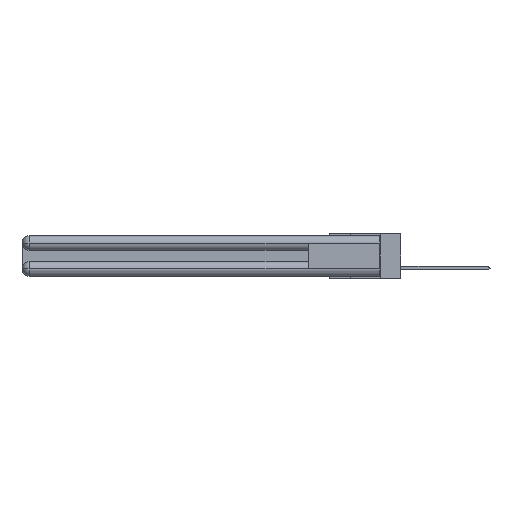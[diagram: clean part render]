
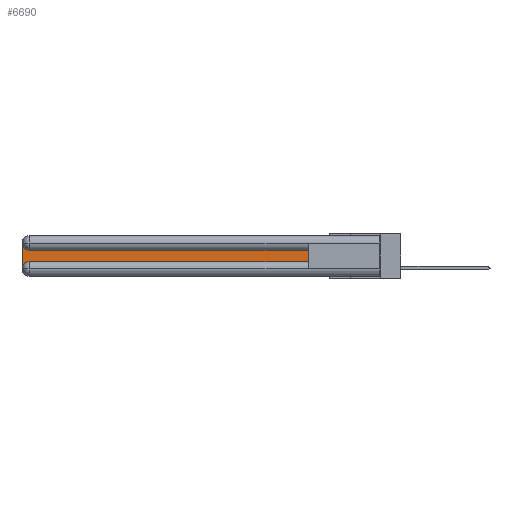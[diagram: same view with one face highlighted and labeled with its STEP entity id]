
A CAD part, left-side view. The second image highlights one B-rep face of the part: STEP entity #6690.
In plain terms, the highlighted planar face has unit normal (-1, 0, 0).
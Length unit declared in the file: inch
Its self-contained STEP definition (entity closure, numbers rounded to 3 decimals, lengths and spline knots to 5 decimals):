
#36 = LINE ( 'NONE', #24860, #5275 ) ;
#130 = EDGE_LOOP ( 'NONE', ( #14637, #1861, #14647, #15981, #6974, #20860 ) ) ;
#1607 = DIRECTION ( 'NONE',  ( 0., 0., -1. ) ) ;
#1852 = CARTESIAN_POINT ( 'NONE',  ( 0.075, 2.94, -0.1225 ) ) ;
#1861 = ORIENTED_EDGE ( 'NONE', *, *, #5569, .T. ) ;
#3278 = VERTEX_POINT ( 'NONE', #14300 ) ;
#3309 = DIRECTION ( 'NONE',  ( 1., 0., 0. ) ) ;
#3866 = DIRECTION ( 'NONE',  ( 0., 1., 0. ) ) ;
#4261 = EDGE_CURVE ( 'NONE', #12910, #3278, #4691, .T. ) ;
#4691 = LINE ( 'NONE', #18431, #27026 ) ;
#4799 = PLANE ( 'NONE',  #11344 ) ;
#4899 = DIRECTION ( 'NONE',  ( 1., 0., 0. ) ) ;
#5275 = VECTOR ( 'NONE', #27114, 39.37008 ) ;
#5452 = VECTOR ( 'NONE', #3866, 39.37008 ) ;
#5569 = EDGE_CURVE ( 'NONE', #20755, #9965, #27325, .T. ) ;
#6690 = ADVANCED_FACE ( 'NONE', ( #25044 ), #4799, .F. ) ;
#6974 = ORIENTED_EDGE ( 'NONE', *, *, #18936, .T. ) ;
#7313 = LINE ( 'NONE', #15847, #16748 ) ;
#8882 = CARTESIAN_POINT ( 'NONE',  ( 0.075, 2.94, -0.2175 ) ) ;
#8989 = CARTESIAN_POINT ( 'NONE',  ( 0.075, 3., -0.2775 ) ) ;
#9965 = VERTEX_POINT ( 'NONE', #11364 ) ;
#11344 = AXIS2_PLACEMENT_3D ( 'NONE', #22553, #4899, #22818 ) ;
#11364 = CARTESIAN_POINT ( 'NONE',  ( 0.075, 3., -0.0625 ) ) ;
#11524 = AXIS2_PLACEMENT_3D ( 'NONE', #18847, #3309, #18940 ) ;
#11785 = DIRECTION ( 'NONE',  ( 0., 0., 1. ) ) ;
#12622 = VERTEX_POINT ( 'NONE', #8989 ) ;
#12910 = VERTEX_POINT ( 'NONE', #16463 ) ;
#14183 = LINE ( 'NONE', #14592, #5452 ) ;
#14300 = CARTESIAN_POINT ( 'NONE',  ( 0.075, 0.6, -0.1225 ) ) ;
#14592 = CARTESIAN_POINT ( 'NONE',  ( 0.075, 0.6, -0.1225 ) ) ;
#14637 = ORIENTED_EDGE ( 'NONE', *, *, #28332, .T. ) ;
#14647 = ORIENTED_EDGE ( 'NONE', *, *, #17142, .T. ) ;
#15257 = CARTESIAN_POINT ( 'NONE',  ( 0.075, 2.94, -0.2775 ) ) ;
#15847 = CARTESIAN_POINT ( 'NONE',  ( 0.075, 0.6, -0.2175 ) ) ;
#15981 = ORIENTED_EDGE ( 'NONE', *, *, #20915, .T. ) ;
#16264 = AXIS2_PLACEMENT_3D ( 'NONE', #15257, #24117, #1607 ) ;
#16463 = CARTESIAN_POINT ( 'NONE',  ( 0.075, 0.6, -0.2175 ) ) ;
#16748 = VECTOR ( 'NONE', #22729, 39.37008 ) ;
#17142 = EDGE_CURVE ( 'NONE', #9965, #12622, #36, .T. ) ;
#18431 = CARTESIAN_POINT ( 'NONE',  ( 0.075, 0.6, -0.2175 ) ) ;
#18847 = CARTESIAN_POINT ( 'NONE',  ( 0.075, 2.94, -0.0625 ) ) ;
#18936 = EDGE_CURVE ( 'NONE', #23937, #12910, #7313, .T. ) ;
#18940 = DIRECTION ( 'NONE',  ( 0., 0., -1. ) ) ;
#20755 = VERTEX_POINT ( 'NONE', #1852 ) ;
#20860 = ORIENTED_EDGE ( 'NONE', *, *, #4261, .T. ) ;
#20915 = EDGE_CURVE ( 'NONE', #12622, #23937, #27099, .T. ) ;
#22553 = CARTESIAN_POINT ( 'NONE',  ( 0.075, 3., -0.1225 ) ) ;
#22729 = DIRECTION ( 'NONE',  ( 0., -1., 0. ) ) ;
#22818 = DIRECTION ( 'NONE',  ( 0., 0., -1. ) ) ;
#23937 = VERTEX_POINT ( 'NONE', #8882 ) ;
#24117 = DIRECTION ( 'NONE',  ( 1., 0., 0. ) ) ;
#24860 = CARTESIAN_POINT ( 'NONE',  ( 0.075, 3., -0.2175 ) ) ;
#25044 = FACE_OUTER_BOUND ( 'NONE', #130, .T. ) ;
#27026 = VECTOR ( 'NONE', #11785, 39.37008 ) ;
#27099 = CIRCLE ( 'NONE', #16264, 0.06 ) ;
#27114 = DIRECTION ( 'NONE',  ( 0., 0., -1. ) ) ;
#27325 = CIRCLE ( 'NONE', #11524, 0.06 ) ;
#28332 = EDGE_CURVE ( 'NONE', #3278, #20755, #14183, .T. ) ;
